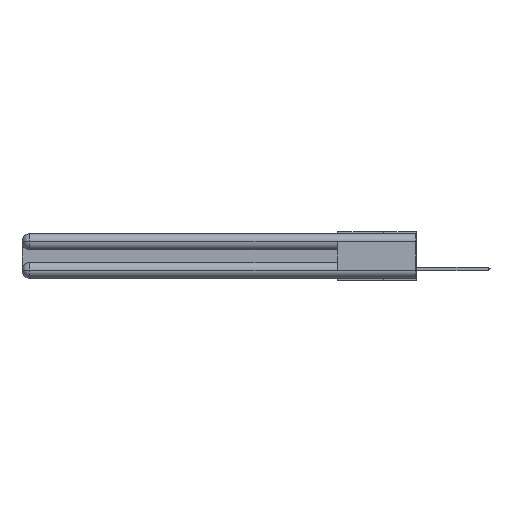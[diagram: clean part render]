
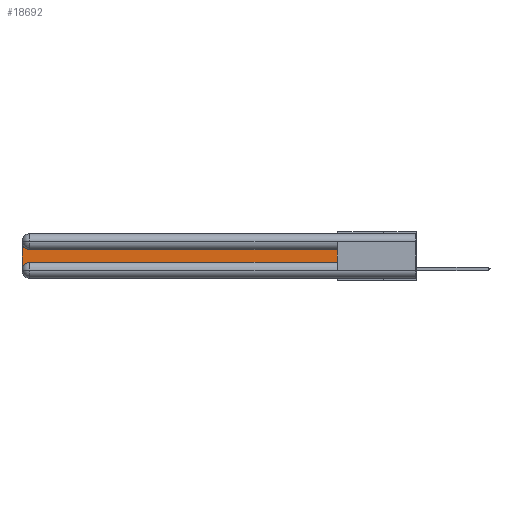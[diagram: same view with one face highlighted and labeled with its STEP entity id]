
A CAD part, left-side view. The second image highlights one B-rep face of the part: STEP entity #18692.
In plain terms, the highlighted planar face has unit normal (-1, 0, 0).
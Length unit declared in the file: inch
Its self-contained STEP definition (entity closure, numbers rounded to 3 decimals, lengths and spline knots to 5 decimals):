
#529 = VECTOR ( 'NONE', #10931, 39.37008 ) ;
#1408 = DIRECTION ( 'NONE',  ( 0., -1., 0. ) ) ;
#1539 = CARTESIAN_POINT ( 'NONE',  ( 0.075, 2.94, -0.0625 ) ) ;
#1732 = LINE ( 'NONE', #2138, #18017 ) ;
#2138 = CARTESIAN_POINT ( 'NONE',  ( 0.075, 0.6, -0.1225 ) ) ;
#2206 = CARTESIAN_POINT ( 'NONE',  ( 0.075, 0.6, -0.1225 ) ) ;
#2615 = CIRCLE ( 'NONE', #5957, 0.06 ) ;
#2643 = VERTEX_POINT ( 'NONE', #25604 ) ;
#2771 = ORIENTED_EDGE ( 'NONE', *, *, #30073, .T. ) ;
#4638 = VERTEX_POINT ( 'NONE', #28618 ) ;
#4648 = CARTESIAN_POINT ( 'NONE',  ( 0.075, 3., -0.1225 ) ) ;
#5957 = AXIS2_PLACEMENT_3D ( 'NONE', #1539, #9045, #16467 ) ;
#7072 = LINE ( 'NONE', #20038, #529 ) ;
#7142 = DIRECTION ( 'NONE',  ( 0., 1., 0. ) ) ;
#8427 = VECTOR ( 'NONE', #31016, 39.37008 ) ;
#8895 = CARTESIAN_POINT ( 'NONE',  ( 0.075, 0.6, -0.2175 ) ) ;
#9045 = DIRECTION ( 'NONE',  ( 1., 0., 0. ) ) ;
#9253 = VERTEX_POINT ( 'NONE', #30791 ) ;
#9861 = DIRECTION ( 'NONE',  ( 1., 0., 0. ) ) ;
#10931 = DIRECTION ( 'NONE',  ( 0., 0., -1. ) ) ;
#11751 = ORIENTED_EDGE ( 'NONE', *, *, #22218, .T. ) ;
#11893 = LINE ( 'NONE', #30892, #8427 ) ;
#13680 = VERTEX_POINT ( 'NONE', #22670 ) ;
#15983 = EDGE_LOOP ( 'NONE', ( #18352, #18325, #11751, #2771, #24018, #30021 ) ) ;
#16310 = LINE ( 'NONE', #8895, #28283 ) ;
#16467 = DIRECTION ( 'NONE',  ( 0., 0., -1. ) ) ;
#17901 = CARTESIAN_POINT ( 'NONE',  ( 0.075, 3., -0.2775 ) ) ;
#18017 = VECTOR ( 'NONE', #7142, 39.37008 ) ;
#18325 = ORIENTED_EDGE ( 'NONE', *, *, #27305, .T. ) ;
#18352 = ORIENTED_EDGE ( 'NONE', *, *, #20717, .T. ) ;
#18598 = AXIS2_PLACEMENT_3D ( 'NONE', #4648, #9861, #31927 ) ;
#18692 = ADVANCED_FACE ( 'NONE', ( #20486 ), #22040, .F. ) ;
#19659 = AXIS2_PLACEMENT_3D ( 'NONE', #21792, #26868, #24309 ) ;
#20038 = CARTESIAN_POINT ( 'NONE',  ( 0.075, 3., -0.2175 ) ) ;
#20486 = FACE_OUTER_BOUND ( 'NONE', #15983, .T. ) ;
#20717 = EDGE_CURVE ( 'NONE', #23523, #9253, #1732, .T. ) ;
#21792 = CARTESIAN_POINT ( 'NONE',  ( 0.075, 2.94, -0.2775 ) ) ;
#22040 = PLANE ( 'NONE',  #18598 ) ;
#22218 = EDGE_CURVE ( 'NONE', #13680, #31536, #7072, .T. ) ;
#22670 = CARTESIAN_POINT ( 'NONE',  ( 0.075, 3., -0.0625 ) ) ;
#22832 = EDGE_CURVE ( 'NONE', #2643, #4638, #16310, .T. ) ;
#23523 = VERTEX_POINT ( 'NONE', #2206 ) ;
#24018 = ORIENTED_EDGE ( 'NONE', *, *, #22832, .T. ) ;
#24309 = DIRECTION ( 'NONE',  ( 0., 0., -1. ) ) ;
#25604 = CARTESIAN_POINT ( 'NONE',  ( 0.075, 2.94, -0.2175 ) ) ;
#26868 = DIRECTION ( 'NONE',  ( 1., 0., 0. ) ) ;
#27305 = EDGE_CURVE ( 'NONE', #9253, #13680, #2615, .T. ) ;
#27521 = EDGE_CURVE ( 'NONE', #4638, #23523, #11893, .T. ) ;
#28283 = VECTOR ( 'NONE', #1408, 39.37008 ) ;
#28618 = CARTESIAN_POINT ( 'NONE',  ( 0.075, 0.6, -0.2175 ) ) ;
#30021 = ORIENTED_EDGE ( 'NONE', *, *, #27521, .T. ) ;
#30073 = EDGE_CURVE ( 'NONE', #31536, #2643, #30300, .T. ) ;
#30300 = CIRCLE ( 'NONE', #19659, 0.06 ) ;
#30791 = CARTESIAN_POINT ( 'NONE',  ( 0.075, 2.94, -0.1225 ) ) ;
#30892 = CARTESIAN_POINT ( 'NONE',  ( 0.075, 0.6, -0.2175 ) ) ;
#31016 = DIRECTION ( 'NONE',  ( 0., 0., 1. ) ) ;
#31536 = VERTEX_POINT ( 'NONE', #17901 ) ;
#31927 = DIRECTION ( 'NONE',  ( 0., 0., -1. ) ) ;
